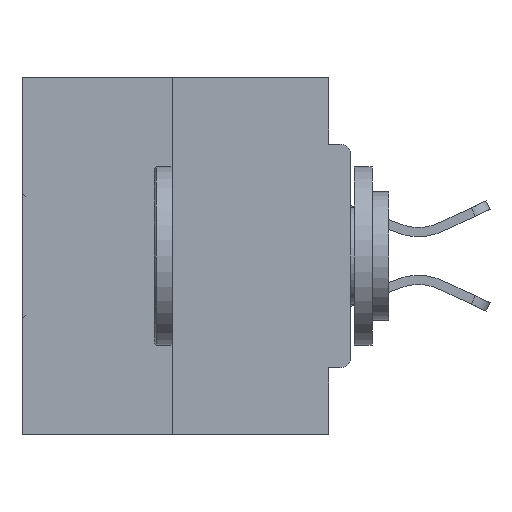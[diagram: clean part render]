
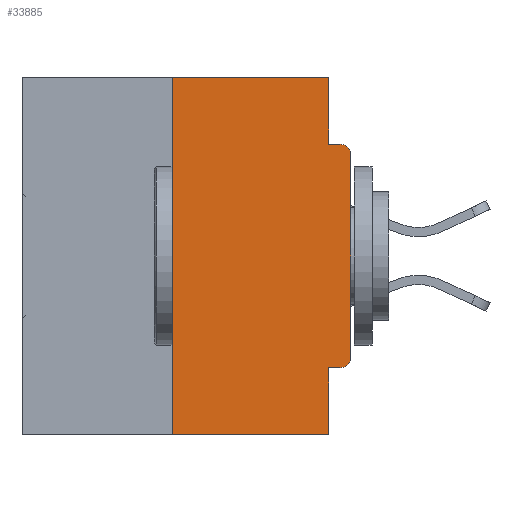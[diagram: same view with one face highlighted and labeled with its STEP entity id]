
A CAD part, left-side view. The second image highlights one B-rep face of the part: STEP entity #33885.
In plain terms, the highlighted planar face has unit normal (-1, 0, 0).
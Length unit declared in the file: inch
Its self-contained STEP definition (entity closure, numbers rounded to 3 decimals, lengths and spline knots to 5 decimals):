
#134 = DIRECTION ( 'NONE',  ( 0., 0., 1. ) ) ;
#447 = LINE ( 'NONE', #41373, #5668 ) ;
#881 = VECTOR ( 'NONE', #4591, 39.37008 ) ;
#933 = LINE ( 'NONE', #12339, #13376 ) ;
#1036 = VECTOR ( 'NONE', #134, 39.37008 ) ;
#1549 = ORIENTED_EDGE ( 'NONE', *, *, #18722, .F. ) ;
#1656 = VERTEX_POINT ( 'NONE', #26118 ) ;
#1933 = CARTESIAN_POINT ( 'NONE',  ( 0., 0., 0. ) ) ;
#2599 = VERTEX_POINT ( 'NONE', #34163 ) ;
#4432 = ORIENTED_EDGE ( 'NONE', *, *, #26917, .F. ) ;
#4459 = DIRECTION ( 'NONE',  ( 0., 0., -1. ) ) ;
#4591 = DIRECTION ( 'NONE',  ( 0., -1., 0. ) ) ;
#5362 = EDGE_CURVE ( 'NONE', #33409, #2599, #15958, .T. ) ;
#5668 = VECTOR ( 'NONE', #31924, 39.37008 ) ;
#6732 = ORIENTED_EDGE ( 'NONE', *, *, #12294, .T. ) ;
#7041 = AXIS2_PLACEMENT_3D ( 'NONE', #40032, #26252, #12988 ) ;
#8615 = CARTESIAN_POINT ( 'NONE',  ( 0., 0.031, 0. ) ) ;
#9543 = ORIENTED_EDGE ( 'NONE', *, *, #27668, .F. ) ;
#9654 = ORIENTED_EDGE ( 'NONE', *, *, #24287, .F. ) ;
#11352 = DIRECTION ( 'NONE',  ( 0., -1., 0. ) ) ;
#11655 = VERTEX_POINT ( 'NONE', #23766 ) ;
#11842 = LINE ( 'NONE', #17604, #881 ) ;
#12294 = EDGE_CURVE ( 'NONE', #11655, #33409, #33302, .T. ) ;
#12317 = CARTESIAN_POINT ( 'NONE',  ( 0., 0.46, 0. ) ) ;
#12339 = CARTESIAN_POINT ( 'NONE',  ( 0., 0.46, -0.5 ) ) ;
#12811 = ORIENTED_EDGE ( 'NONE', *, *, #14713, .F. ) ;
#12968 = ORIENTED_EDGE ( 'NONE', *, *, #14576, .T. ) ;
#12988 = DIRECTION ( 'NONE',  ( 0., 0., -1. ) ) ;
#13363 = AXIS2_PLACEMENT_3D ( 'NONE', #12317, #18643, #41987 ) ;
#13376 = VECTOR ( 'NONE', #22558, 39.37008 ) ;
#14576 = EDGE_CURVE ( 'NONE', #33366, #1656, #933, .T. ) ;
#14713 = EDGE_CURVE ( 'NONE', #18238, #2599, #11842, .T. ) ;
#15819 = VECTOR ( 'NONE', #4459, 39.37008 ) ;
#15958 = CIRCLE ( 'NONE', #35284, 0.015 ) ;
#16118 = ORIENTED_EDGE ( 'NONE', *, *, #5362, .T. ) ;
#16216 = EDGE_CURVE ( 'NONE', #42158, #11655, #22821, .T. ) ;
#16561 = CARTESIAN_POINT ( 'NONE',  ( 0., 0.25, 0. ) ) ;
#17209 = ORIENTED_EDGE ( 'NONE', *, *, #42551, .F. ) ;
#17604 = CARTESIAN_POINT ( 'NONE',  ( 0., 0., -0.0935 ) ) ;
#17890 = EDGE_LOOP ( 'NONE', ( #1549, #4432, #12968, #9543, #9654, #18813, #6732, #16118, #12811, #17209 ) ) ;
#18238 = VERTEX_POINT ( 'NONE', #39347 ) ;
#18643 = DIRECTION ( 'NONE',  ( 1., 0., 0. ) ) ;
#18722 = EDGE_CURVE ( 'NONE', #25929, #20478, #36508, .T. ) ;
#18780 = PLANE ( 'NONE',  #13363 ) ;
#18813 = ORIENTED_EDGE ( 'NONE', *, *, #16216, .T. ) ;
#18831 = CARTESIAN_POINT ( 'NONE',  ( 0., 0.031, -0.4065 ) ) ;
#18856 = VERTEX_POINT ( 'NONE', #18831 ) ;
#19122 = CARTESIAN_POINT ( 'NONE',  ( 0., 0.25, -0.5 ) ) ;
#20478 = VERTEX_POINT ( 'NONE', #8615 ) ;
#20955 = CARTESIAN_POINT ( 'NONE',  ( 0., 0.031, 0. ) ) ;
#21916 = DIRECTION ( 'NONE',  ( 0., 0., -1. ) ) ;
#22558 = DIRECTION ( 'NONE',  ( 0., -1., 0. ) ) ;
#22821 = CIRCLE ( 'NONE', #7041, 0.015 ) ;
#23766 = CARTESIAN_POINT ( 'NONE',  ( 0., 0., -0.3915 ) ) ;
#23904 = VECTOR ( 'NONE', #28229, 39.37008 ) ;
#24287 = EDGE_CURVE ( 'NONE', #42158, #18856, #37949, .T. ) ;
#25233 = CARTESIAN_POINT ( 'NONE',  ( 0., 0.015, -0.1085 ) ) ;
#25929 = VERTEX_POINT ( 'NONE', #16561 ) ;
#26118 = CARTESIAN_POINT ( 'NONE',  ( 0., 0.031, -0.5 ) ) ;
#26252 = DIRECTION ( 'NONE',  ( -1., 0., 0. ) ) ;
#26917 = EDGE_CURVE ( 'NONE', #33366, #25929, #32641, .T. ) ;
#27668 = EDGE_CURVE ( 'NONE', #18856, #1656, #447, .T. ) ;
#28229 = DIRECTION ( 'NONE',  ( 0., 1., 0. ) ) ;
#31098 = CARTESIAN_POINT ( 'NONE',  ( 0., 0., -0.4065 ) ) ;
#31924 = DIRECTION ( 'NONE',  ( 0., 0., -1. ) ) ;
#32025 = DIRECTION ( 'NONE',  ( 0., 0., 1. ) ) ;
#32289 = VECTOR ( 'NONE', #32025, 39.37008 ) ;
#32351 = LINE ( 'NONE', #20955, #15819 ) ;
#32438 = CARTESIAN_POINT ( 'NONE',  ( 0., 0., -0.1085 ) ) ;
#32641 = LINE ( 'NONE', #33264, #1036 ) ;
#32912 = VECTOR ( 'NONE', #11352, 39.37008 ) ;
#33264 = CARTESIAN_POINT ( 'NONE',  ( 0., 0.25, 0. ) ) ;
#33302 = LINE ( 'NONE', #1933, #32289 ) ;
#33366 = VERTEX_POINT ( 'NONE', #19122 ) ;
#33409 = VERTEX_POINT ( 'NONE', #32438 ) ;
#33885 = ADVANCED_FACE ( 'NONE', ( #34532 ), #18780, .F. ) ;
#34163 = CARTESIAN_POINT ( 'NONE',  ( 0., 0.015, -0.0935 ) ) ;
#34532 = FACE_OUTER_BOUND ( 'NONE', #17890, .T. ) ;
#35235 = DIRECTION ( 'NONE',  ( -1., 0., 0. ) ) ;
#35284 = AXIS2_PLACEMENT_3D ( 'NONE', #25233, #35235, #21916 ) ;
#36508 = LINE ( 'NONE', #40892, #32912 ) ;
#37949 = LINE ( 'NONE', #31098, #23904 ) ;
#39347 = CARTESIAN_POINT ( 'NONE',  ( 0., 0.031, -0.0935 ) ) ;
#40032 = CARTESIAN_POINT ( 'NONE',  ( 0., 0.015, -0.3915 ) ) ;
#40892 = CARTESIAN_POINT ( 'NONE',  ( 0., 0.46, 0. ) ) ;
#41182 = CARTESIAN_POINT ( 'NONE',  ( 0., 0.015, -0.4065 ) ) ;
#41373 = CARTESIAN_POINT ( 'NONE',  ( 0., 0.031, -0.5 ) ) ;
#41987 = DIRECTION ( 'NONE',  ( 0., 0., -1. ) ) ;
#42158 = VERTEX_POINT ( 'NONE', #41182 ) ;
#42551 = EDGE_CURVE ( 'NONE', #20478, #18238, #32351, .T. ) ;
